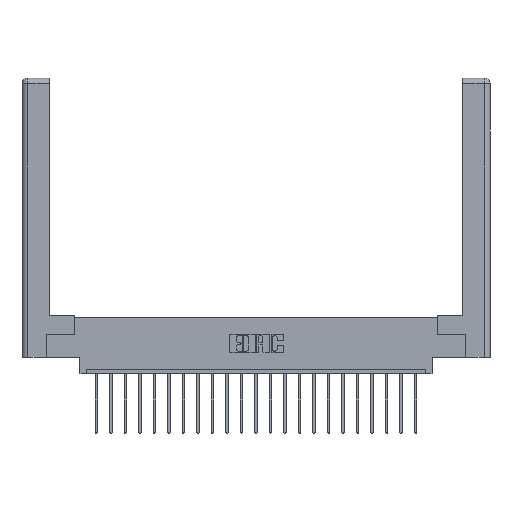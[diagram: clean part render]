
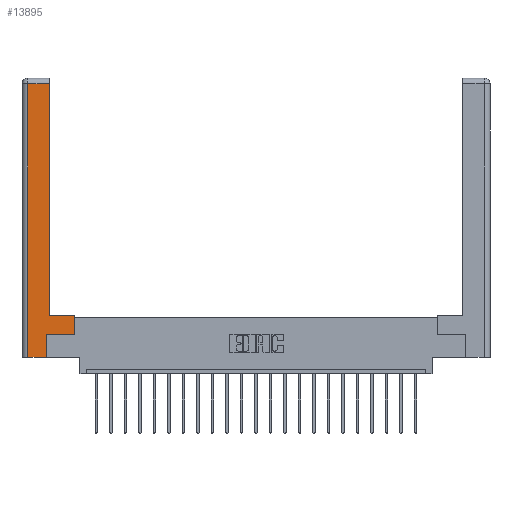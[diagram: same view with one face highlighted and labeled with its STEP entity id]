
A CAD part, top view. The second image highlights one B-rep face of the part: STEP entity #13895.
In plain terms, the highlighted planar face has unit normal (0, 0, 1).
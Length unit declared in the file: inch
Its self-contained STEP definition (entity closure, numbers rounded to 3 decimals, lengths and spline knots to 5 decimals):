
#47 = DIRECTION ( 'NONE',  ( 0., -1., 0. ) ) ;
#102 = DIRECTION ( 'NONE',  ( 0., 1., 0. ) ) ;
#175 = VECTOR ( 'NONE', #9100, 39.37008 ) ;
#331 = VERTEX_POINT ( 'NONE', #9136 ) ;
#359 = DIRECTION ( 'NONE',  ( -1., 0., 0. ) ) ;
#470 = VERTEX_POINT ( 'NONE', #9588 ) ;
#810 = AXIS2_PLACEMENT_3D ( 'NONE', #20675, #10335, #359 ) ;
#1571 = EDGE_CURVE ( 'NONE', #3056, #16465, #19689, .T. ) ;
#1683 = VECTOR ( 'NONE', #47, 39.37008 ) ;
#1840 = DIRECTION ( 'NONE',  ( -1., 0., 0. ) ) ;
#2106 = CARTESIAN_POINT ( 'NONE',  ( 0.565, 0.245, 0. ) ) ;
#2348 = CARTESIAN_POINT ( 'NONE',  ( 0.565, 0.45, 0. ) ) ;
#2779 = CARTESIAN_POINT ( 'NONE',  ( 0.0615, 0., 0. ) ) ;
#3056 = VERTEX_POINT ( 'NONE', #21834 ) ;
#3247 = VECTOR ( 'NONE', #3567, 39.37008 ) ;
#3567 = DIRECTION ( 'NONE',  ( -1., 0., 0. ) ) ;
#4459 = DIRECTION ( 'NONE',  ( 0., 1., 0. ) ) ;
#4517 = ORIENTED_EDGE ( 'NONE', *, *, #11464, .T. ) ;
#4865 = LINE ( 'NONE', #15591, #13792 ) ;
#5072 = CARTESIAN_POINT ( 'NONE',  ( 0.0615, 2.94, 0. ) ) ;
#5476 = VERTEX_POINT ( 'NONE', #7765 ) ;
#5598 = LINE ( 'NONE', #2106, #19127 ) ;
#6554 = ORIENTED_EDGE ( 'NONE', *, *, #1571, .T. ) ;
#6942 = LINE ( 'NONE', #17403, #175 ) ;
#7102 = VERTEX_POINT ( 'NONE', #16963 ) ;
#7765 = CARTESIAN_POINT ( 'NONE',  ( 0.295, 2.94, 0. ) ) ;
#7945 = ORIENTED_EDGE ( 'NONE', *, *, #15027, .T. ) ;
#8153 = EDGE_CURVE ( 'NONE', #14553, #17596, #14666, .T. ) ;
#9100 = DIRECTION ( 'NONE',  ( 0., 1., 0. ) ) ;
#9136 = CARTESIAN_POINT ( 'NONE',  ( 0.265, 0.245, 0. ) ) ;
#9245 = ORIENTED_EDGE ( 'NONE', *, *, #18713, .T. ) ;
#9588 = CARTESIAN_POINT ( 'NONE',  ( 0.295, 0.45, 0. ) ) ;
#9917 = VECTOR ( 'NONE', #11459, 39.37008 ) ;
#10335 = DIRECTION ( 'NONE',  ( 0., 0., -1. ) ) ;
#10474 = VECTOR ( 'NONE', #4459, 39.37008 ) ;
#10520 = CARTESIAN_POINT ( 'NONE',  ( 0.0615, 2.94, 0. ) ) ;
#11003 = EDGE_CURVE ( 'NONE', #16465, #470, #4865, .T. ) ;
#11240 = FACE_OUTER_BOUND ( 'NONE', #21899, .T. ) ;
#11459 = DIRECTION ( 'NONE',  ( 1., 0., 0. ) ) ;
#11464 = EDGE_CURVE ( 'NONE', #5476, #14553, #12441, .T. ) ;
#12441 = LINE ( 'NONE', #10520, #3247 ) ;
#12896 = LINE ( 'NONE', #17383, #17771 ) ;
#13020 = EDGE_CURVE ( 'NONE', #470, #5476, #12896, .T. ) ;
#13703 = EDGE_CURVE ( 'NONE', #7102, #331, #6942, .T. ) ;
#13792 = VECTOR ( 'NONE', #1840, 39.37008 ) ;
#13895 = ADVANCED_FACE ( 'NONE', ( #11240 ), #22297, .F. ) ;
#14183 = DIRECTION ( 'NONE',  ( 1., 0., 0. ) ) ;
#14209 = LINE ( 'NONE', #18200, #9917 ) ;
#14553 = VERTEX_POINT ( 'NONE', #5072 ) ;
#14666 = LINE ( 'NONE', #17629, #1683 ) ;
#15027 = EDGE_CURVE ( 'NONE', #17596, #7102, #14209, .T. ) ;
#15591 = CARTESIAN_POINT ( 'NONE',  ( 0.295, 0.45, 0. ) ) ;
#15668 = ORIENTED_EDGE ( 'NONE', *, *, #8153, .T. ) ;
#16465 = VERTEX_POINT ( 'NONE', #2348 ) ;
#16509 = CARTESIAN_POINT ( 'NONE',  ( 0.565, 0.45, 0. ) ) ;
#16963 = CARTESIAN_POINT ( 'NONE',  ( 0.265, 0., 0. ) ) ;
#17383 = CARTESIAN_POINT ( 'NONE',  ( 0.295, 3., 0. ) ) ;
#17403 = CARTESIAN_POINT ( 'NONE',  ( 0.265, 0.245, 0. ) ) ;
#17596 = VERTEX_POINT ( 'NONE', #2779 ) ;
#17629 = CARTESIAN_POINT ( 'NONE',  ( 0.0615, 0., 0. ) ) ;
#17771 = VECTOR ( 'NONE', #102, 39.37008 ) ;
#18200 = CARTESIAN_POINT ( 'NONE',  ( 0.265, 0., 0. ) ) ;
#18713 = EDGE_CURVE ( 'NONE', #331, #3056, #5598, .T. ) ;
#18890 = ORIENTED_EDGE ( 'NONE', *, *, #13703, .T. ) ;
#19127 = VECTOR ( 'NONE', #14183, 39.37008 ) ;
#19689 = LINE ( 'NONE', #16509, #10474 ) ;
#20675 = CARTESIAN_POINT ( 'NONE',  ( 0., 0., 0. ) ) ;
#20914 = ORIENTED_EDGE ( 'NONE', *, *, #11003, .T. ) ;
#21834 = CARTESIAN_POINT ( 'NONE',  ( 0.565, 0.245, 0. ) ) ;
#21899 = EDGE_LOOP ( 'NONE', ( #22123, #4517, #15668, #7945, #18890, #9245, #6554, #20914 ) ) ;
#22123 = ORIENTED_EDGE ( 'NONE', *, *, #13020, .T. ) ;
#22297 = PLANE ( 'NONE',  #810 ) ;
